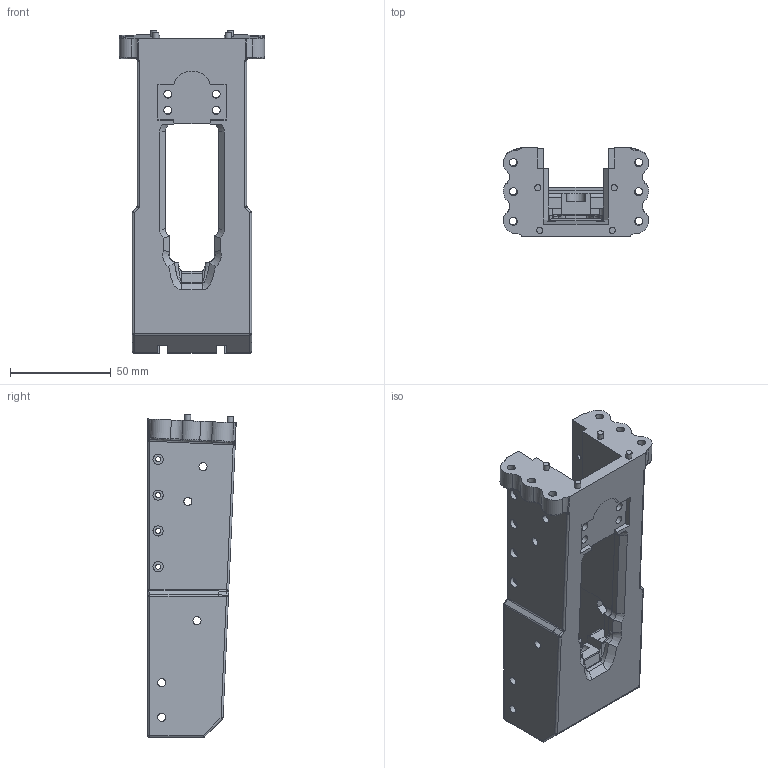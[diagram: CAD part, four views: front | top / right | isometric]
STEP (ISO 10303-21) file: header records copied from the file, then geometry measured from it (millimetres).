
FILE_DESCRIPTION(/* description */ (''),/* implementation_level */ '2;1');
FILE_NAME(/* name */ 'Plastikov v0.9 Front Receiver.stp',/* time_stamp */ '2019-12-22T15:33:01-06:00',/* author */ ('johne'),/* organization */ (''),/* preprocessor_version */ 'ST-DEVELOPER v18',/* originating_system */ 'Autodesk Inventor 2020',/* authorisation */ '');
FILE_SCHEMA (('AUTOMOTIVE_DESIGN { 1 0 10303 214 3 1 1 }'));
Length unit declared in the file: millimetre
Products named in the file (1): Plastikov Trial Front Recevier v6 redo
Bounding box: 72.2 x 43.88 x 160.38 mm (x, y, z)
Volume: 186790.4 mm3; surface area: 45485.4 mm2
Topology: 1 solids, 1 shells, 348 faces, 903 edges, 568 vertices
Faces by surface type: plane 166, cylinder 108, bspline 39, torus 16, sphere 13, cone 6
Full cylindrical faces by diameter (mm): 2.5 x8, 3 x4, 4 x20, 4.05 x1, 5.08 x8
Entity records: 11945 total; most frequent: CARTESIAN_POINT 3329, ORIENTED_EDGE 1790, DIRECTION 1745, EDGE_CURVE 895, AXIS2_PLACEMENT_3D 608, VERTEX_POINT 568, LINE 529, VECTOR 529
